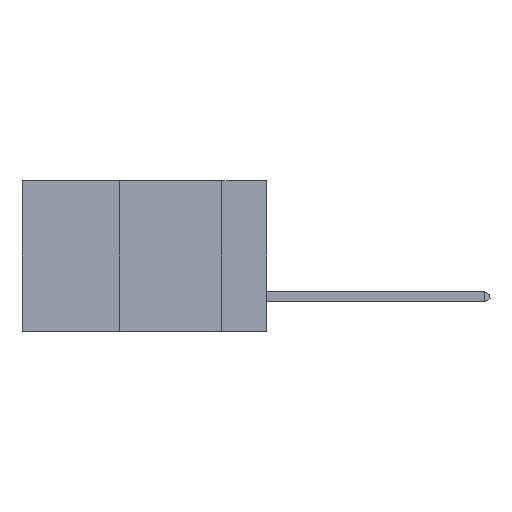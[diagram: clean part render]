
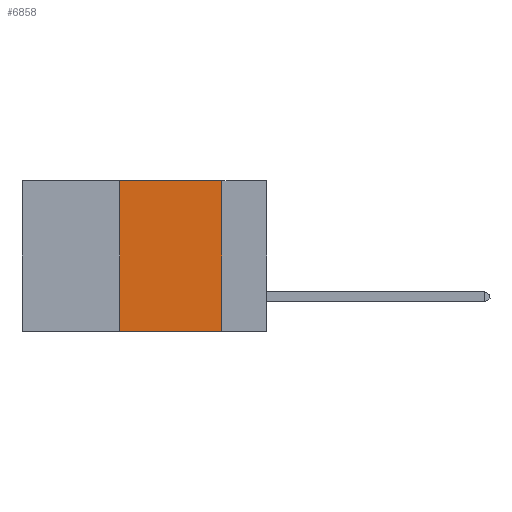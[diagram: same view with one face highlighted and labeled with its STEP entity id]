
A CAD part, left-side view. The second image highlights one B-rep face of the part: STEP entity #6858.
In plain terms, the highlighted planar face has unit normal (-1, 0, 0).
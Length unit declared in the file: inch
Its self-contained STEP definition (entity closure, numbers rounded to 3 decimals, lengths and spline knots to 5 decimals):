
#668 = DIRECTION ( 'NONE',  ( 0., 0., -1. ) ) ;
#1786 = EDGE_LOOP ( 'NONE', ( #6468, #9580, #4001, #8906 ) ) ;
#1814 = FACE_OUTER_BOUND ( 'NONE', #1786, .T. ) ;
#2464 = DIRECTION ( 'NONE',  ( 0., -1., 0. ) ) ;
#2937 = LINE ( 'NONE', #4968, #12500 ) ;
#4001 = ORIENTED_EDGE ( 'NONE', *, *, #12110, .F. ) ;
#4342 = CARTESIAN_POINT ( 'NONE',  ( 0., 0.36, 0. ) ) ;
#4968 = CARTESIAN_POINT ( 'NONE',  ( 0., 0.6, 0. ) ) ;
#5134 = VECTOR ( 'NONE', #668, 39.37008 ) ;
#5285 = DIRECTION ( 'NONE',  ( 0., 0., 1. ) ) ;
#5390 = AXIS2_PLACEMENT_3D ( 'NONE', #12041, #11904, #11903 ) ;
#5820 = VERTEX_POINT ( 'NONE', #6462 ) ;
#6052 = VECTOR ( 'NONE', #5285, 39.37008 ) ;
#6112 = EDGE_CURVE ( 'NONE', #10036, #5820, #2937, .T. ) ;
#6349 = LINE ( 'NONE', #4342, #6052 ) ;
#6462 = CARTESIAN_POINT ( 'NONE',  ( 0., 0.11, 0. ) ) ;
#6468 = ORIENTED_EDGE ( 'NONE', *, *, #11757, .F. ) ;
#6858 = ADVANCED_FACE ( 'NONE', ( #1814 ), #11917, .F. ) ;
#7154 = EDGE_CURVE ( 'NONE', #12283, #7385, #10780, .T. ) ;
#7385 = VERTEX_POINT ( 'NONE', #8530 ) ;
#7586 = CARTESIAN_POINT ( 'NONE',  ( 0., 0.36, -0.37 ) ) ;
#8270 = VECTOR ( 'NONE', #9916, 39.37008 ) ;
#8530 = CARTESIAN_POINT ( 'NONE',  ( 0., 0.11, -0.37 ) ) ;
#8581 = CARTESIAN_POINT ( 'NONE',  ( 0., 0.11, 0. ) ) ;
#8906 = ORIENTED_EDGE ( 'NONE', *, *, #7154, .T. ) ;
#9580 = ORIENTED_EDGE ( 'NONE', *, *, #6112, .F. ) ;
#9916 = DIRECTION ( 'NONE',  ( 0., -1., 0. ) ) ;
#10036 = VERTEX_POINT ( 'NONE', #10443 ) ;
#10062 = CARTESIAN_POINT ( 'NONE',  ( 0., 0.6, -0.37 ) ) ;
#10271 = LINE ( 'NONE', #8581, #5134 ) ;
#10443 = CARTESIAN_POINT ( 'NONE',  ( 0., 0.36, 0. ) ) ;
#10780 = LINE ( 'NONE', #10062, #8270 ) ;
#11757 = EDGE_CURVE ( 'NONE', #5820, #7385, #10271, .T. ) ;
#11903 = DIRECTION ( 'NONE',  ( 0., 0., -1. ) ) ;
#11904 = DIRECTION ( 'NONE',  ( 1., 0., 0. ) ) ;
#11917 = PLANE ( 'NONE',  #5390 ) ;
#12041 = CARTESIAN_POINT ( 'NONE',  ( 0., 0.6, 0. ) ) ;
#12110 = EDGE_CURVE ( 'NONE', #12283, #10036, #6349, .T. ) ;
#12283 = VERTEX_POINT ( 'NONE', #7586 ) ;
#12500 = VECTOR ( 'NONE', #2464, 39.37008 ) ;
